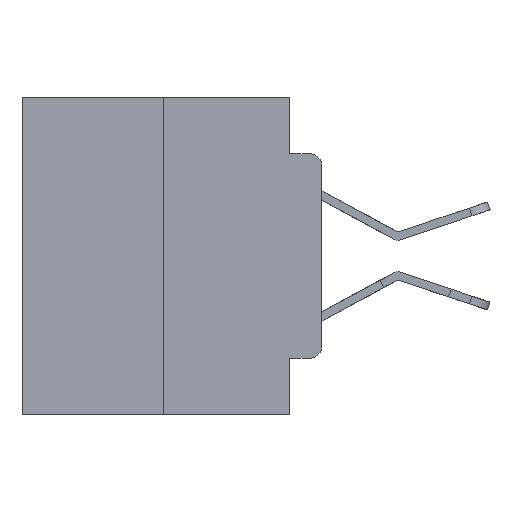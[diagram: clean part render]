
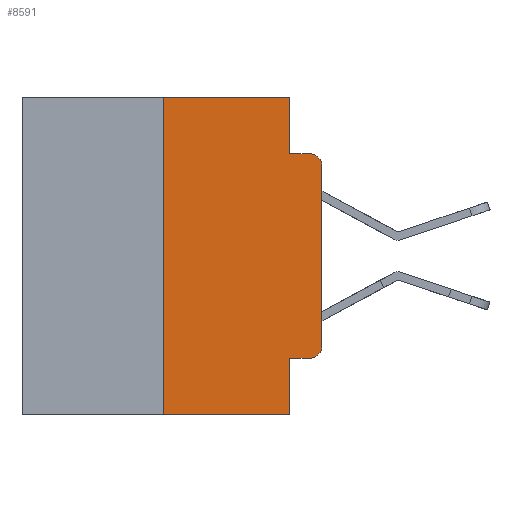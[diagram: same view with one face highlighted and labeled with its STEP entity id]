
A CAD part, left-side view. The second image highlights one B-rep face of the part: STEP entity #8591.
In plain terms, the highlighted planar face has unit normal (-1, 0, 0).
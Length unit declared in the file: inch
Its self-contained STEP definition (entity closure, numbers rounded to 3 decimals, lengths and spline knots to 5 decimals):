
#187 = DIRECTION ( 'NONE',  ( 0., 0., -1. ) ) ;
#302 = AXIS2_PLACEMENT_3D ( 'NONE', #26051, #13236, #187 ) ;
#539 = CARTESIAN_POINT ( 'NONE',  ( 0., 0.473, 0. ) ) ;
#610 = EDGE_CURVE ( 'NONE', #19293, #17591, #13820, .T. ) ;
#804 = DIRECTION ( 'NONE',  ( 0., -1., 0. ) ) ;
#1074 = DIRECTION ( 'NONE',  ( 0., 0., -1. ) ) ;
#1244 = AXIS2_PLACEMENT_3D ( 'NONE', #11630, #26561, #13747 ) ;
#1301 = CARTESIAN_POINT ( 'NONE',  ( 0., 0.25, -0.5 ) ) ;
#1321 = ORIENTED_EDGE ( 'NONE', *, *, #12965, .F. ) ;
#1768 = CARTESIAN_POINT ( 'NONE',  ( 0., 0., 0. ) ) ;
#2102 = EDGE_CURVE ( 'NONE', #23978, #2115, #5339, .T. ) ;
#2115 = VERTEX_POINT ( 'NONE', #25871 ) ;
#2913 = CARTESIAN_POINT ( 'NONE',  ( 0., 0.25, 0. ) ) ;
#2964 = ORIENTED_EDGE ( 'NONE', *, *, #18679, .T. ) ;
#4214 = VECTOR ( 'NONE', #17891, 39.37008 ) ;
#4409 = CARTESIAN_POINT ( 'NONE',  ( 0., 0.051, 0. ) ) ;
#4521 = CARTESIAN_POINT ( 'NONE',  ( 0., 0.02, -0.0885 ) ) ;
#4528 = CARTESIAN_POINT ( 'NONE',  ( 0., 0.051, 0. ) ) ;
#5339 = LINE ( 'NONE', #4409, #16742 ) ;
#5340 = ORIENTED_EDGE ( 'NONE', *, *, #9001, .F. ) ;
#6200 = VECTOR ( 'NONE', #22230, 39.37008 ) ;
#6202 = ORIENTED_EDGE ( 'NONE', *, *, #8775, .T. ) ;
#6404 = ORIENTED_EDGE ( 'NONE', *, *, #7169, .F. ) ;
#6679 = ORIENTED_EDGE ( 'NONE', *, *, #610, .T. ) ;
#7169 = EDGE_CURVE ( 'NONE', #20625, #11814, #23276, .T. ) ;
#7171 = LINE ( 'NONE', #9556, #12159 ) ;
#7518 = VECTOR ( 'NONE', #804, 39.37008 ) ;
#7689 = CIRCLE ( 'NONE', #1244, 0.02 ) ;
#8386 = CARTESIAN_POINT ( 'NONE',  ( 0., 0.051, -0.0885 ) ) ;
#8570 = CARTESIAN_POINT ( 'NONE',  ( 0., 0.051, -0.4115 ) ) ;
#8591 = ADVANCED_FACE ( 'NONE', ( #27878 ), #9851, .F. ) ;
#8775 = EDGE_CURVE ( 'NONE', #16403, #22169, #13165, .T. ) ;
#9001 = EDGE_CURVE ( 'NONE', #19293, #20124, #7171, .T. ) ;
#9556 = CARTESIAN_POINT ( 'NONE',  ( 0., 0.051, 0. ) ) ;
#9851 = PLANE ( 'NONE',  #20363 ) ;
#10485 = DIRECTION ( 'NONE',  ( 0., -1., 0. ) ) ;
#11530 = CARTESIAN_POINT ( 'NONE',  ( 0., 0., -0.1085 ) ) ;
#11573 = EDGE_LOOP ( 'NONE', ( #6202, #20409, #15239, #24750, #1321, #6404, #2964, #5340, #6679, #25295 ) ) ;
#11621 = EDGE_CURVE ( 'NONE', #17591, #16403, #24796, .T. ) ;
#11630 = CARTESIAN_POINT ( 'NONE',  ( 0., 0.02, -0.1085 ) ) ;
#11685 = DIRECTION ( 'NONE',  ( 0., 0., -1. ) ) ;
#11814 = VERTEX_POINT ( 'NONE', #18095 ) ;
#12159 = VECTOR ( 'NONE', #11685, 39.37008 ) ;
#12965 = EDGE_CURVE ( 'NONE', #11814, #23978, #16306, .T. ) ;
#13151 = VECTOR ( 'NONE', #19702, 39.37008 ) ;
#13165 = LINE ( 'NONE', #1768, #23231 ) ;
#13236 = DIRECTION ( 'NONE',  ( -1., 0., 0. ) ) ;
#13747 = DIRECTION ( 'NONE',  ( 0., 0., -1. ) ) ;
#13820 = LINE ( 'NONE', #8570, #13151 ) ;
#14104 = DIRECTION ( 'NONE',  ( 1., 0., 0. ) ) ;
#15164 = CARTESIAN_POINT ( 'NONE',  ( 0., 0., -0.3915 ) ) ;
#15239 = ORIENTED_EDGE ( 'NONE', *, *, #19453, .F. ) ;
#15766 = VECTOR ( 'NONE', #10485, 39.37008 ) ;
#16306 = LINE ( 'NONE', #539, #4214 ) ;
#16403 = VERTEX_POINT ( 'NONE', #15164 ) ;
#16742 = VECTOR ( 'NONE', #19428, 39.37008 ) ;
#17591 = VERTEX_POINT ( 'NONE', #27638 ) ;
#17891 = DIRECTION ( 'NONE',  ( 0., -1., 0. ) ) ;
#18095 = CARTESIAN_POINT ( 'NONE',  ( 0., 0.25, 0. ) ) ;
#18679 = EDGE_CURVE ( 'NONE', #20625, #20124, #23875, .T. ) ;
#19062 = DIRECTION ( 'NONE',  ( 0., 0., 1. ) ) ;
#19293 = VERTEX_POINT ( 'NONE', #24793 ) ;
#19428 = DIRECTION ( 'NONE',  ( 0., 0., -1. ) ) ;
#19453 = EDGE_CURVE ( 'NONE', #2115, #26902, #20794, .T. ) ;
#19702 = DIRECTION ( 'NONE',  ( 0., -1., 0. ) ) ;
#20124 = VERTEX_POINT ( 'NONE', #25570 ) ;
#20363 = AXIS2_PLACEMENT_3D ( 'NONE', #26909, #14104, #1074 ) ;
#20409 = ORIENTED_EDGE ( 'NONE', *, *, #22177, .T. ) ;
#20625 = VERTEX_POINT ( 'NONE', #1301 ) ;
#20794 = LINE ( 'NONE', #8386, #15766 ) ;
#22169 = VERTEX_POINT ( 'NONE', #11530 ) ;
#22177 = EDGE_CURVE ( 'NONE', #22169, #26902, #7689, .T. ) ;
#22230 = DIRECTION ( 'NONE',  ( 0., 0., 1. ) ) ;
#23231 = VECTOR ( 'NONE', #19062, 39.37008 ) ;
#23276 = LINE ( 'NONE', #2913, #6200 ) ;
#23875 = LINE ( 'NONE', #26657, #7518 ) ;
#23978 = VERTEX_POINT ( 'NONE', #4528 ) ;
#24750 = ORIENTED_EDGE ( 'NONE', *, *, #2102, .F. ) ;
#24793 = CARTESIAN_POINT ( 'NONE',  ( 0., 0.051, -0.4115 ) ) ;
#24796 = CIRCLE ( 'NONE', #302, 0.02 ) ;
#25295 = ORIENTED_EDGE ( 'NONE', *, *, #11621, .T. ) ;
#25570 = CARTESIAN_POINT ( 'NONE',  ( 0., 0.051, -0.5 ) ) ;
#25871 = CARTESIAN_POINT ( 'NONE',  ( 0., 0.051, -0.0885 ) ) ;
#26051 = CARTESIAN_POINT ( 'NONE',  ( 0., 0.02, -0.3915 ) ) ;
#26561 = DIRECTION ( 'NONE',  ( -1., 0., 0. ) ) ;
#26657 = CARTESIAN_POINT ( 'NONE',  ( 0., 0.473, -0.5 ) ) ;
#26902 = VERTEX_POINT ( 'NONE', #4521 ) ;
#26909 = CARTESIAN_POINT ( 'NONE',  ( 0., 0.473, 0. ) ) ;
#27638 = CARTESIAN_POINT ( 'NONE',  ( 0., 0.02, -0.4115 ) ) ;
#27878 = FACE_OUTER_BOUND ( 'NONE', #11573, .T. ) ;
